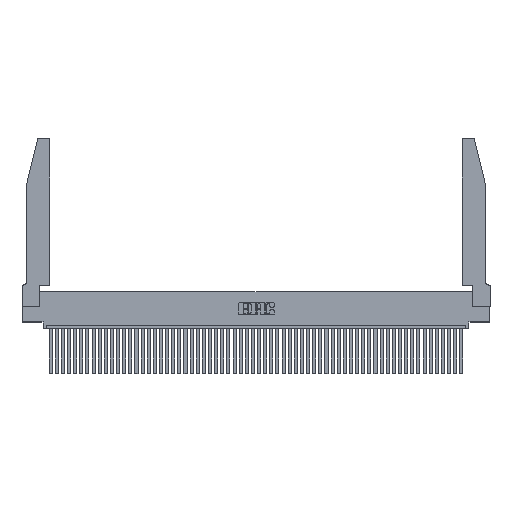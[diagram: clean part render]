
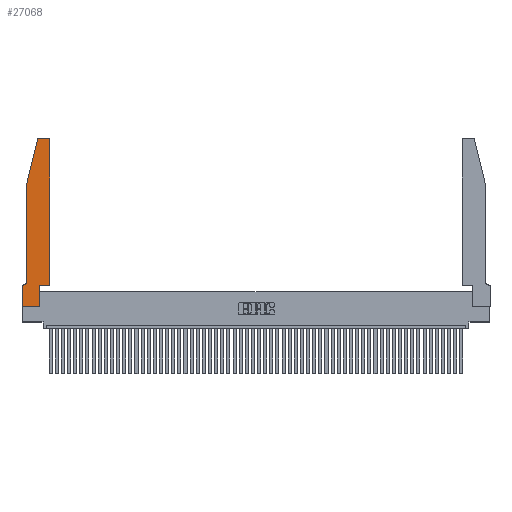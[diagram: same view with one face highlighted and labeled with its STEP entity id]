
A CAD part, top view. The second image highlights one B-rep face of the part: STEP entity #27068.
In plain terms, the highlighted planar face has unit normal (0, 0, 1).
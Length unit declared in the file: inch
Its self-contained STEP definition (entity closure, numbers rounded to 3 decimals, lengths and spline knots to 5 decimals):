
#201 = CARTESIAN_POINT ( 'NONE',  ( 0.0755, 2., 0.37 ) ) ;
#581 = VERTEX_POINT ( 'NONE', #11574 ) ;
#585 = VERTEX_POINT ( 'NONE', #19718 ) ;
#1073 = VECTOR ( 'NONE', #24017, 39.37008 ) ;
#1332 = DIRECTION ( 'NONE',  ( 0., 0., 1. ) ) ;
#2066 = VERTEX_POINT ( 'NONE', #14087 ) ;
#2591 = CARTESIAN_POINT ( 'NONE',  ( 0.25487, 2.72718, 0.37 ) ) ;
#4642 = DIRECTION ( 'NONE',  ( -0.239, -0.971, 0. ) ) ;
#5237 = AXIS2_PLACEMENT_3D ( 'NONE', #12391, #24915, #12914 ) ;
#5426 = VERTEX_POINT ( 'NONE', #46203 ) ;
#5429 = VECTOR ( 'NONE', #12452, 39.37008 ) ;
#5555 = CARTESIAN_POINT ( 'NONE',  ( 0., 0., 0.37 ) ) ;
#5894 = LINE ( 'NONE', #35894, #47613 ) ;
#6309 = CARTESIAN_POINT ( 'NONE',  ( 0.284, 2.75, 0.37 ) ) ;
#6946 = ORIENTED_EDGE ( 'NONE', *, *, #7122, .T. ) ;
#7122 = EDGE_CURVE ( 'NONE', #38840, #581, #38911, .T. ) ;
#8137 = VERTEX_POINT ( 'NONE', #34059 ) ;
#9087 = DIRECTION ( 'NONE',  ( 0., 1., 0. ) ) ;
#9593 = CARTESIAN_POINT ( 'NONE',  ( 0.2865, 0.35, 0.37 ) ) ;
#9889 = ORIENTED_EDGE ( 'NONE', *, *, #31440, .T. ) ;
#10300 = LINE ( 'NONE', #10502, #49480 ) ;
#10502 = CARTESIAN_POINT ( 'NONE',  ( 0.0755, 0.35, 0.37 ) ) ;
#10529 = EDGE_LOOP ( 'NONE', ( #12532, #34925, #23154, #51703, #9889, #34679, #39379, #48976, #45263, #30889, #6946, #14182 ) ) ;
#10534 = CARTESIAN_POINT ( 'NONE',  ( 0., 0.35, 0.37 ) ) ;
#10666 = DIRECTION ( 'NONE',  ( -1., 0., 0. ) ) ;
#11574 = CARTESIAN_POINT ( 'NONE',  ( 0.4505, 2.72, 0.37 ) ) ;
#11668 = DIRECTION ( 'NONE',  ( 1., 0., 0. ) ) ;
#11926 = CIRCLE ( 'NONE', #5237, 0.07 ) ;
#12267 = DIRECTION ( 'NONE',  ( 0., -1., 0. ) ) ;
#12391 = CARTESIAN_POINT ( 'NONE',  ( 0.0055, 0.42, 0.37 ) ) ;
#12452 = DIRECTION ( 'NONE',  ( -1., 0., 0. ) ) ;
#12532 = ORIENTED_EDGE ( 'NONE', *, *, #27020, .T. ) ;
#12841 = CARTESIAN_POINT ( 'NONE',  ( 0., 0.35, 0.37 ) ) ;
#12914 = DIRECTION ( 'NONE',  ( -1., 0., 0. ) ) ;
#13168 = VECTOR ( 'NONE', #9087, 39.37008 ) ;
#13435 = EDGE_CURVE ( 'NONE', #36803, #35681, #43553, .T. ) ;
#14087 = CARTESIAN_POINT ( 'NONE',  ( 0.2865, 0., 0.37 ) ) ;
#14182 = ORIENTED_EDGE ( 'NONE', *, *, #36990, .T. ) ;
#15676 = CARTESIAN_POINT ( 'NONE',  ( 0.4205, 2.72, 0.37 ) ) ;
#16331 = EDGE_CURVE ( 'NONE', #585, #2066, #5894, .T. ) ;
#18547 = CARTESIAN_POINT ( 'NONE',  ( 0.0755, 2., 0.37 ) ) ;
#18729 = EDGE_CURVE ( 'NONE', #35681, #31775, #51746, .T. ) ;
#18973 = DIRECTION ( 'NONE',  ( 0., 1., 0. ) ) ;
#19718 = CARTESIAN_POINT ( 'NONE',  ( 0., 0., 0.37 ) ) ;
#20295 = VECTOR ( 'NONE', #12267, 39.37008 ) ;
#22871 = LINE ( 'NONE', #36486, #20295 ) ;
#23154 = ORIENTED_EDGE ( 'NONE', *, *, #18729, .T. ) ;
#23618 = DIRECTION ( 'NONE',  ( 0., 0., 1. ) ) ;
#23859 = CARTESIAN_POINT ( 'NONE',  ( 0.4205, 2.75, 0.37 ) ) ;
#24017 = DIRECTION ( 'NONE',  ( 1., 0., 0. ) ) ;
#24031 = EDGE_CURVE ( 'NONE', #2066, #28571, #29588, .T. ) ;
#24798 = DIRECTION ( 'NONE',  ( 0., 0., 1. ) ) ;
#24915 = DIRECTION ( 'NONE',  ( 0., 0., -1. ) ) ;
#25021 = AXIS2_PLACEMENT_3D ( 'NONE', #12841, #24798, #42484 ) ;
#25575 = CARTESIAN_POINT ( 'NONE',  ( 0.284, 2.72, 0.37 ) ) ;
#27020 = EDGE_CURVE ( 'NONE', #48559, #36803, #47801, .T. ) ;
#27068 = ADVANCED_FACE ( 'NONE', ( #28846 ), #41173, .T. ) ;
#27261 = CARTESIAN_POINT ( 'NONE',  ( 0.4505, 0.35, 0.37 ) ) ;
#28571 = VERTEX_POINT ( 'NONE', #31322 ) ;
#28846 = FACE_OUTER_BOUND ( 'NONE', #10529, .T. ) ;
#28907 = CARTESIAN_POINT ( 'NONE',  ( 0.4505, 0.35, 0.37 ) ) ;
#29588 = LINE ( 'NONE', #9593, #13168 ) ;
#29635 = DIRECTION ( 'NONE',  ( 1., 0., 0. ) ) ;
#30889 = ORIENTED_EDGE ( 'NONE', *, *, #50859, .T. ) ;
#31322 = CARTESIAN_POINT ( 'NONE',  ( 0.2865, 0.35, 0.37 ) ) ;
#31440 = EDGE_CURVE ( 'NONE', #5426, #8137, #11926, .T. ) ;
#31775 = VERTEX_POINT ( 'NONE', #18547 ) ;
#32814 = EDGE_CURVE ( 'NONE', #31775, #5426, #22871, .T. ) ;
#34000 = DIRECTION ( 'NONE',  ( 0., -1., 0. ) ) ;
#34059 = CARTESIAN_POINT ( 'NONE',  ( 0.0055, 0.35, 0.37 ) ) ;
#34448 = VERTEX_POINT ( 'NONE', #10534 ) ;
#34679 = ORIENTED_EDGE ( 'NONE', *, *, #37537, .T. ) ;
#34925 = ORIENTED_EDGE ( 'NONE', *, *, #13435, .T. ) ;
#35681 = VERTEX_POINT ( 'NONE', #2591 ) ;
#35894 = CARTESIAN_POINT ( 'NONE',  ( 0., 0., 0.37 ) ) ;
#36486 = CARTESIAN_POINT ( 'NONE',  ( 0.0755, 2., 0.37 ) ) ;
#36668 = CARTESIAN_POINT ( 'NONE',  ( 0.2605, 2.75, 0.37 ) ) ;
#36803 = VERTEX_POINT ( 'NONE', #6309 ) ;
#36990 = EDGE_CURVE ( 'NONE', #581, #48559, #43855, .T. ) ;
#37537 = EDGE_CURVE ( 'NONE', #8137, #34448, #10300, .T. ) ;
#38290 = VECTOR ( 'NONE', #34000, 39.37008 ) ;
#38840 = VERTEX_POINT ( 'NONE', #28907 ) ;
#38911 = LINE ( 'NONE', #27261, #46505 ) ;
#39379 = ORIENTED_EDGE ( 'NONE', *, *, #39710, .T. ) ;
#39710 = EDGE_CURVE ( 'NONE', #34448, #585, #42083, .T. ) ;
#41173 = PLANE ( 'NONE',  #25021 ) ;
#41595 = AXIS2_PLACEMENT_3D ( 'NONE', #15676, #23618, #51315 ) ;
#42083 = LINE ( 'NONE', #5555, #38290 ) ;
#42484 = DIRECTION ( 'NONE',  ( 1., 0., 0. ) ) ;
#43553 = CIRCLE ( 'NONE', #52392, 0.03 ) ;
#43855 = CIRCLE ( 'NONE', #41595, 0.03 ) ;
#44317 = CARTESIAN_POINT ( 'NONE',  ( 0.4505, 0.35, 0.37 ) ) ;
#44829 = VECTOR ( 'NONE', #4642, 39.37008 ) ;
#45263 = ORIENTED_EDGE ( 'NONE', *, *, #24031, .T. ) ;
#46203 = CARTESIAN_POINT ( 'NONE',  ( 0.0755, 0.42, 0.37 ) ) ;
#46505 = VECTOR ( 'NONE', #18973, 39.37008 ) ;
#47613 = VECTOR ( 'NONE', #11668, 39.37008 ) ;
#47801 = LINE ( 'NONE', #36668, #5429 ) ;
#48494 = LINE ( 'NONE', #44317, #1073 ) ;
#48559 = VERTEX_POINT ( 'NONE', #23859 ) ;
#48976 = ORIENTED_EDGE ( 'NONE', *, *, #16331, .T. ) ;
#49480 = VECTOR ( 'NONE', #10666, 39.37008 ) ;
#50859 = EDGE_CURVE ( 'NONE', #28571, #38840, #48494, .T. ) ;
#51315 = DIRECTION ( 'NONE',  ( 1., 0., 0. ) ) ;
#51703 = ORIENTED_EDGE ( 'NONE', *, *, #32814, .T. ) ;
#51746 = LINE ( 'NONE', #201, #44829 ) ;
#52392 = AXIS2_PLACEMENT_3D ( 'NONE', #25575, #1332, #29635 ) ;
